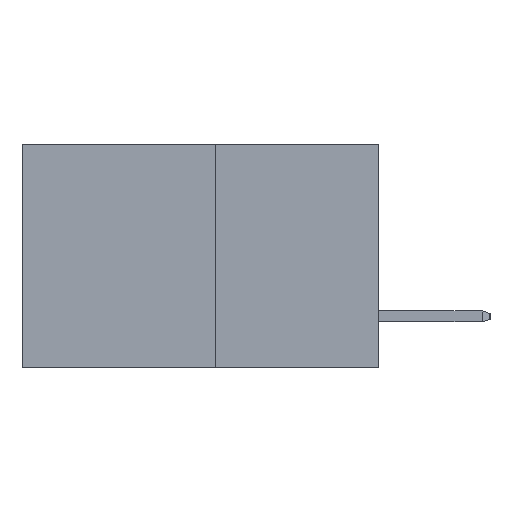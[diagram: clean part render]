
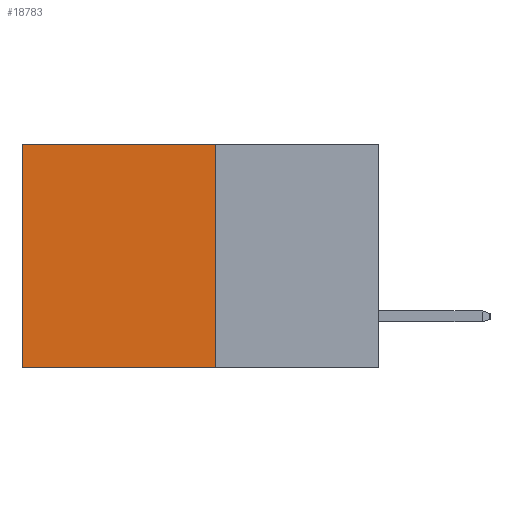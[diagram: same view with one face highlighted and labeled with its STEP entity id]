
A CAD part, left-side view. The second image highlights one B-rep face of the part: STEP entity #18783.
In plain terms, the highlighted planar face has unit normal (-1, 0, 0).
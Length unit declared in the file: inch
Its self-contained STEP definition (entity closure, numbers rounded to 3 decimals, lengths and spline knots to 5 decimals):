
#80 = EDGE_CURVE ( 'NONE', #25282, #1137, #6873, .T. ) ;
#875 = VECTOR ( 'NONE', #17227, 39.37008 ) ;
#1063 = DIRECTION ( 'NONE',  ( 0., 1., 0. ) ) ;
#1137 = VERTEX_POINT ( 'NONE', #25300 ) ;
#2353 = DIRECTION ( 'NONE',  ( 0., 1., 0. ) ) ;
#2482 = ORIENTED_EDGE ( 'NONE', *, *, #21506, .F. ) ;
#2594 = DIRECTION ( 'NONE',  ( 1., 0., 0. ) ) ;
#3173 = LINE ( 'NONE', #13468, #19984 ) ;
#3304 = CARTESIAN_POINT ( 'NONE',  ( 0.277, 0.27, -0.37 ) ) ;
#4676 = ORIENTED_EDGE ( 'NONE', *, *, #10152, .F. ) ;
#6873 = LINE ( 'NONE', #17713, #875 ) ;
#9719 = CARTESIAN_POINT ( 'NONE',  ( 0.277, 0.27, -0.37 ) ) ;
#9945 = EDGE_CURVE ( 'NONE', #16386, #25282, #3173, .T. ) ;
#10027 = CARTESIAN_POINT ( 'NONE',  ( 0.277, 0.27, -0.37 ) ) ;
#10152 = EDGE_CURVE ( 'NONE', #16386, #18335, #25323, .T. ) ;
#10287 = EDGE_LOOP ( 'NONE', ( #21316, #2482, #4676, #10704 ) ) ;
#10704 = ORIENTED_EDGE ( 'NONE', *, *, #9945, .T. ) ;
#11536 = PLANE ( 'NONE',  #24661 ) ;
#11945 = DIRECTION ( 'NONE',  ( 0., 0., -1. ) ) ;
#13468 = CARTESIAN_POINT ( 'NONE',  ( 0.277, 0.27, 0. ) ) ;
#15862 = CARTESIAN_POINT ( 'NONE',  ( 0.277, 0.27, -0.37 ) ) ;
#16386 = VERTEX_POINT ( 'NONE', #20829 ) ;
#16815 = VECTOR ( 'NONE', #1063, 39.37008 ) ;
#17227 = DIRECTION ( 'NONE',  ( 0., 0., -1. ) ) ;
#17713 = CARTESIAN_POINT ( 'NONE',  ( 0.277, 0.59, -0.37 ) ) ;
#17979 = DIRECTION ( 'NONE',  ( 0., 0., -1. ) ) ;
#18335 = VERTEX_POINT ( 'NONE', #3304 ) ;
#18783 = ADVANCED_FACE ( 'NONE', ( #27617 ), #11536, .F. ) ;
#19632 = VECTOR ( 'NONE', #11945, 39.37008 ) ;
#19984 = VECTOR ( 'NONE', #2353, 39.37008 ) ;
#20829 = CARTESIAN_POINT ( 'NONE',  ( 0.277, 0.27, 0. ) ) ;
#21316 = ORIENTED_EDGE ( 'NONE', *, *, #80, .T. ) ;
#21506 = EDGE_CURVE ( 'NONE', #18335, #1137, #22489, .T. ) ;
#22489 = LINE ( 'NONE', #10027, #16815 ) ;
#24661 = AXIS2_PLACEMENT_3D ( 'NONE', #15862, #2594, #17979 ) ;
#25282 = VERTEX_POINT ( 'NONE', #25519 ) ;
#25300 = CARTESIAN_POINT ( 'NONE',  ( 0.277, 0.59, -0.37 ) ) ;
#25323 = LINE ( 'NONE', #9719, #19632 ) ;
#25519 = CARTESIAN_POINT ( 'NONE',  ( 0.277, 0.59, 0. ) ) ;
#27617 = FACE_OUTER_BOUND ( 'NONE', #10287, .T. ) ;
